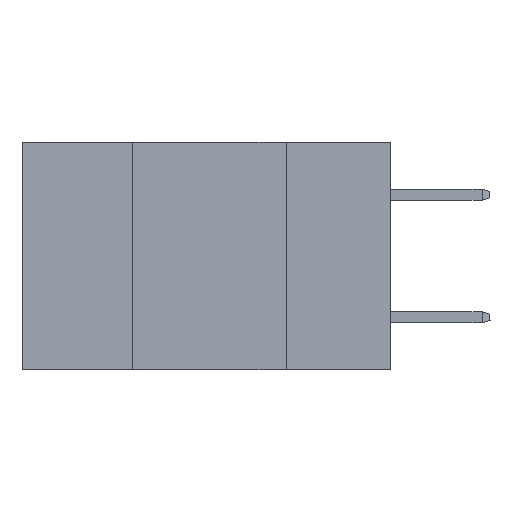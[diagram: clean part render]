
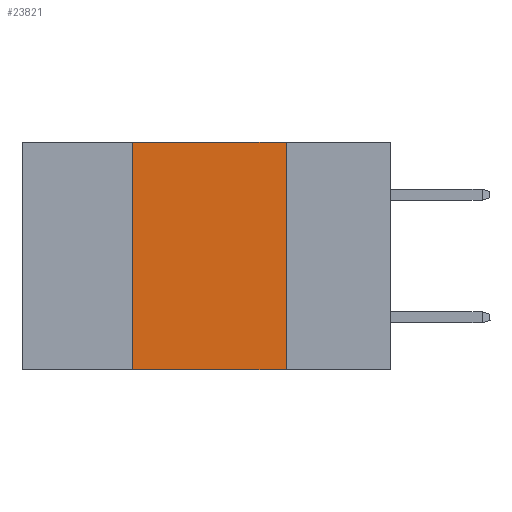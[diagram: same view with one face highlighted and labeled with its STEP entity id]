
A CAD part, left-side view. The second image highlights one B-rep face of the part: STEP entity #23821.
In plain terms, the highlighted planar face has unit normal (-1, 0, 0).
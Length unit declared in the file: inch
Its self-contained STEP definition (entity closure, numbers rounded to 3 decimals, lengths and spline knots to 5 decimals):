
#332 = CARTESIAN_POINT ( 'NONE',  ( 0., 0.6, -0.37 ) ) ;
#464 = EDGE_CURVE ( 'NONE', #20659, #8174, #25747, .T. ) ;
#492 = ORIENTED_EDGE ( 'NONE', *, *, #464, .F. ) ;
#2944 = CARTESIAN_POINT ( 'NONE',  ( 0., 0.42, 0. ) ) ;
#4940 = VECTOR ( 'NONE', #13429, 39.37008 ) ;
#8174 = VERTEX_POINT ( 'NONE', #29804 ) ;
#8291 = DIRECTION ( 'NONE',  ( 0., 0., -1. ) ) ;
#9928 = VERTEX_POINT ( 'NONE', #29518 ) ;
#12512 = VERTEX_POINT ( 'NONE', #19486 ) ;
#13429 = DIRECTION ( 'NONE',  ( 0., 0., -1. ) ) ;
#13637 = LINE ( 'NONE', #33371, #4940 ) ;
#14361 = DIRECTION ( 'NONE',  ( 0., -1., 0. ) ) ;
#16042 = LINE ( 'NONE', #332, #41014 ) ;
#16788 = EDGE_CURVE ( 'NONE', #9928, #12512, #13637, .T. ) ;
#18031 = CARTESIAN_POINT ( 'NONE',  ( 0., 0.6, 0. ) ) ;
#19486 = CARTESIAN_POINT ( 'NONE',  ( 0., 0.17, -0.37 ) ) ;
#20057 = ORIENTED_EDGE ( 'NONE', *, *, #38454, .T. ) ;
#20659 = VERTEX_POINT ( 'NONE', #38176 ) ;
#20834 = ORIENTED_EDGE ( 'NONE', *, *, #16788, .F. ) ;
#21087 = VECTOR ( 'NONE', #14361, 39.37008 ) ;
#21123 = EDGE_CURVE ( 'NONE', #8174, #9928, #34934, .T. ) ;
#23668 = PLANE ( 'NONE',  #24347 ) ;
#23814 = CARTESIAN_POINT ( 'NONE',  ( 0., 0.6, 0. ) ) ;
#23821 = ADVANCED_FACE ( 'NONE', ( #33665 ), #23668, .F. ) ;
#24347 = AXIS2_PLACEMENT_3D ( 'NONE', #23814, #30388, #8291 ) ;
#25747 = LINE ( 'NONE', #2944, #39011 ) ;
#28172 = ORIENTED_EDGE ( 'NONE', *, *, #21123, .F. ) ;
#28619 = DIRECTION ( 'NONE',  ( 0., 0., 1. ) ) ;
#29518 = CARTESIAN_POINT ( 'NONE',  ( 0., 0.17, 0. ) ) ;
#29804 = CARTESIAN_POINT ( 'NONE',  ( 0., 0.42, 0. ) ) ;
#30388 = DIRECTION ( 'NONE',  ( 1., 0., 0. ) ) ;
#33371 = CARTESIAN_POINT ( 'NONE',  ( 0., 0.17, 0. ) ) ;
#33665 = FACE_OUTER_BOUND ( 'NONE', #41291, .T. ) ;
#34934 = LINE ( 'NONE', #18031, #21087 ) ;
#36243 = DIRECTION ( 'NONE',  ( 0., -1., 0. ) ) ;
#38176 = CARTESIAN_POINT ( 'NONE',  ( 0., 0.42, -0.37 ) ) ;
#38454 = EDGE_CURVE ( 'NONE', #20659, #12512, #16042, .T. ) ;
#39011 = VECTOR ( 'NONE', #28619, 39.37008 ) ;
#41014 = VECTOR ( 'NONE', #36243, 39.37008 ) ;
#41291 = EDGE_LOOP ( 'NONE', ( #20834, #28172, #492, #20057 ) ) ;
